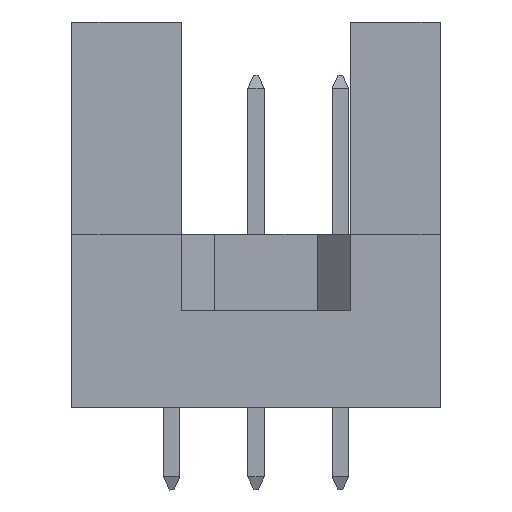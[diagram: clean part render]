
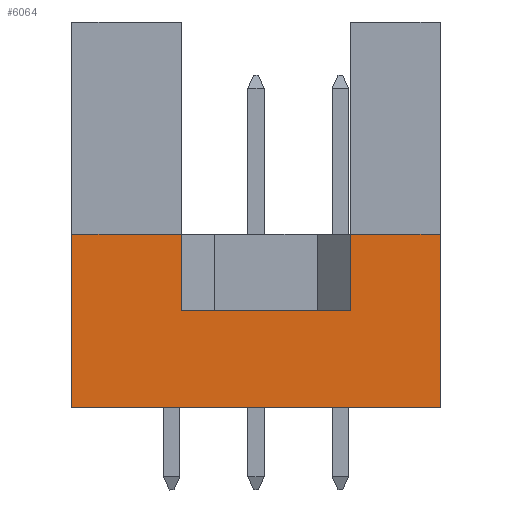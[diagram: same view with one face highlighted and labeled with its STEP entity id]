
A CAD part, left-side view. The second image highlights one B-rep face of the part: STEP entity #6064.
In plain terms, the highlighted planar face has unit normal (-1, 0, 0).
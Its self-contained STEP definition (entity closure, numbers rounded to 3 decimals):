
#42 = AXIS2_PLACEMENT_3D ( 'NONE', #66, #5918, #2162 ) ;
#66 = CARTESIAN_POINT ( 'NONE',  ( -19.9, 11.1, 0. ) ) ;
#264 = VERTEX_POINT ( 'NONE', #1810 ) ;
#265 = DIRECTION ( 'NONE',  ( 0., 0., 1. ) ) ;
#411 = EDGE_CURVE ( 'NONE', #2045, #2637, #5092, .T. ) ;
#607 = DIRECTION ( 'NONE',  ( 0., 0., 1. ) ) ;
#750 = VERTEX_POINT ( 'NONE', #5251 ) ;
#915 = ORIENTED_EDGE ( 'NONE', *, *, #1278, .T. ) ;
#921 = VECTOR ( 'NONE', #3238, 1000. ) ;
#1139 = LINE ( 'NONE', #4249, #921 ) ;
#1228 = ORIENTED_EDGE ( 'NONE', *, *, #411, .T. ) ;
#1278 = EDGE_CURVE ( 'NONE', #1785, #5700, #3484, .T. ) ;
#1342 = EDGE_CURVE ( 'NONE', #2045, #264, #6713, .T. ) ;
#1368 = VECTOR ( 'NONE', #607, 1000. ) ;
#1465 = DIRECTION ( 'NONE',  ( 0., -1., 0. ) ) ;
#1604 = LINE ( 'NONE', #5956, #6695 ) ;
#1667 = EDGE_CURVE ( 'NONE', #4306, #750, #3951, .T. ) ;
#1747 = DIRECTION ( 'NONE',  ( 0., -1., 0. ) ) ;
#1785 = VERTEX_POINT ( 'NONE', #5612 ) ;
#1796 = CARTESIAN_POINT ( 'NONE',  ( -19.9, 11.1, 5.2 ) ) ;
#1810 = CARTESIAN_POINT ( 'NONE',  ( -19.9, 2.71, 2.9 ) ) ;
#1942 = DIRECTION ( 'NONE',  ( 0., -1., 0. ) ) ;
#2045 = VERTEX_POINT ( 'NONE', #4761 ) ;
#2162 = DIRECTION ( 'NONE',  ( 0., 0., -1. ) ) ;
#2292 = CARTESIAN_POINT ( 'NONE',  ( -19.9, 11.1, 0. ) ) ;
#2636 = VECTOR ( 'NONE', #3037, 1000. ) ;
#2637 = VERTEX_POINT ( 'NONE', #4204 ) ;
#2853 = EDGE_LOOP ( 'NONE', ( #5218, #1228, #3265, #3579, #915, #3394, #5185, #5790 ) ) ;
#2971 = VECTOR ( 'NONE', #1942, 1000. ) ;
#2977 = VECTOR ( 'NONE', #1465, 1000. ) ;
#3037 = DIRECTION ( 'NONE',  ( 0., -1., 0. ) ) ;
#3214 = VECTOR ( 'NONE', #265, 1000. ) ;
#3238 = DIRECTION ( 'NONE',  ( 0., 0., 1. ) ) ;
#3265 = ORIENTED_EDGE ( 'NONE', *, *, #5969, .F. ) ;
#3394 = ORIENTED_EDGE ( 'NONE', *, *, #6580, .T. ) ;
#3433 = VERTEX_POINT ( 'NONE', #4022 ) ;
#3484 = LINE ( 'NONE', #6184, #2636 ) ;
#3511 = LINE ( 'NONE', #2292, #4355 ) ;
#3579 = ORIENTED_EDGE ( 'NONE', *, *, #6092, .F. ) ;
#3791 = FACE_OUTER_BOUND ( 'NONE', #2853, .T. ) ;
#3951 = LINE ( 'NONE', #1796, #2977 ) ;
#4022 = CARTESIAN_POINT ( 'NONE',  ( -19.9, 11.1, 5.2 ) ) ;
#4204 = CARTESIAN_POINT ( 'NONE',  ( -19.9, 7.79, 5.2 ) ) ;
#4249 = CARTESIAN_POINT ( 'NONE',  ( -19.9, 0., 0. ) ) ;
#4306 = VERTEX_POINT ( 'NONE', #4876 ) ;
#4355 = VECTOR ( 'NONE', #5000, 1000. ) ;
#4646 = CARTESIAN_POINT ( 'NONE',  ( -19.9, 7.79, 2.9 ) ) ;
#4761 = CARTESIAN_POINT ( 'NONE',  ( -19.9, 7.79, 2.9 ) ) ;
#4876 = CARTESIAN_POINT ( 'NONE',  ( -19.9, 2.71, 5.2 ) ) ;
#5000 = DIRECTION ( 'NONE',  ( 0., 0., 1. ) ) ;
#5092 = LINE ( 'NONE', #6153, #3214 ) ;
#5185 = ORIENTED_EDGE ( 'NONE', *, *, #1667, .F. ) ;
#5218 = ORIENTED_EDGE ( 'NONE', *, *, #1342, .F. ) ;
#5251 = CARTESIAN_POINT ( 'NONE',  ( -19.9, 0., 5.2 ) ) ;
#5299 = LINE ( 'NONE', #5342, #1368 ) ;
#5342 = CARTESIAN_POINT ( 'NONE',  ( -19.9, 2.71, 2.9 ) ) ;
#5504 = CARTESIAN_POINT ( 'NONE',  ( -19.9, 0., 0. ) ) ;
#5612 = CARTESIAN_POINT ( 'NONE',  ( -19.9, 11.1, 0. ) ) ;
#5700 = VERTEX_POINT ( 'NONE', #5504 ) ;
#5790 = ORIENTED_EDGE ( 'NONE', *, *, #6397, .F. ) ;
#5918 = DIRECTION ( 'NONE',  ( 1., 0., 0. ) ) ;
#5956 = CARTESIAN_POINT ( 'NONE',  ( -19.9, 11.1, 5.2 ) ) ;
#5969 = EDGE_CURVE ( 'NONE', #3433, #2637, #1604, .T. ) ;
#5989 = PLANE ( 'NONE',  #42 ) ;
#6064 = ADVANCED_FACE ( 'NONE', ( #3791 ), #5989, .F. ) ;
#6092 = EDGE_CURVE ( 'NONE', #1785, #3433, #3511, .T. ) ;
#6153 = CARTESIAN_POINT ( 'NONE',  ( -19.9, 7.79, 2.9 ) ) ;
#6184 = CARTESIAN_POINT ( 'NONE',  ( -19.9, 11.1, 0. ) ) ;
#6397 = EDGE_CURVE ( 'NONE', #264, #4306, #5299, .T. ) ;
#6580 = EDGE_CURVE ( 'NONE', #5700, #750, #1139, .T. ) ;
#6695 = VECTOR ( 'NONE', #1747, 1000. ) ;
#6713 = LINE ( 'NONE', #4646, #2971 ) ;
